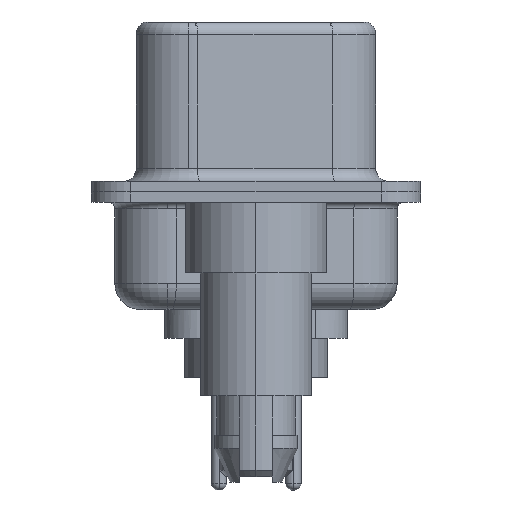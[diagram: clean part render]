
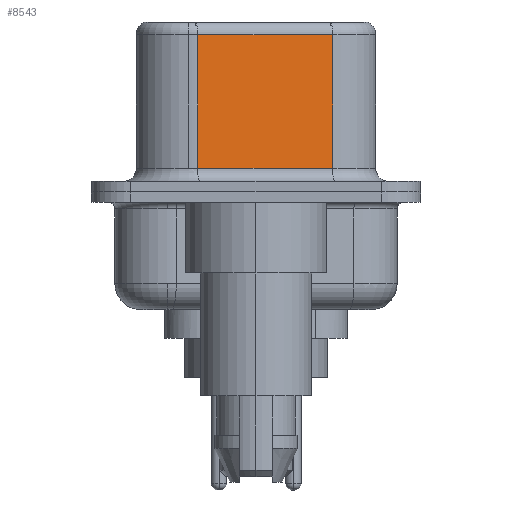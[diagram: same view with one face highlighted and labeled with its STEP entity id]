
A CAD part, left-side view. The second image highlights one B-rep face of the part: STEP entity #8543.
In plain terms, the highlighted planar face has unit normal (-0.985, -0.174, 0).
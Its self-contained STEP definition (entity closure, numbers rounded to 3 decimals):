
#245 = ORIENTED_EDGE ( 'NONE', *, *, #7230, .F. ) ;
#458 = PLANE ( 'NONE',  #13292 ) ;
#678 = VERTEX_POINT ( 'NONE', #21382 ) ;
#1195 = DIRECTION ( 'NONE',  ( 0., 0., -1. ) ) ;
#2364 = CARTESIAN_POINT ( 'NONE',  ( 4.58, -2.927, 6.02 ) ) ;
#2941 = LINE ( 'NONE', #6671, #22758 ) ;
#3120 = VECTOR ( 'NONE', #1195, 1000. ) ;
#4083 = ORIENTED_EDGE ( 'NONE', *, *, #16837, .T. ) ;
#4992 = EDGE_CURVE ( 'NONE', #20967, #20509, #14270, .T. ) ;
#5473 = DIRECTION ( 'NONE',  ( 0., 0., -1. ) ) ;
#6671 = CARTESIAN_POINT ( 'NONE',  ( 4.58, -2.927, 6.52 ) ) ;
#7089 = LINE ( 'NONE', #2364, #20712 ) ;
#7230 = EDGE_CURVE ( 'NONE', #678, #20509, #2941, .T. ) ;
#8213 = LINE ( 'NONE', #23555, #3120 ) ;
#8543 = ADVANCED_FACE ( 'NONE', ( #9182 ), #458, .F. ) ;
#9182 = FACE_OUTER_BOUND ( 'NONE', #14926, .T. ) ;
#9293 = VECTOR ( 'NONE', #22135, 1000. ) ;
#9952 = CARTESIAN_POINT ( 'NONE',  ( 4.58, -2.927, 6.52 ) ) ;
#10033 = DIRECTION ( 'NONE',  ( 0.985, 0.174, 0. ) ) ;
#10299 = EDGE_CURVE ( 'NONE', #10715, #20967, #8213, .T. ) ;
#10715 = VERTEX_POINT ( 'NONE', #14763 ) ;
#13292 = AXIS2_PLACEMENT_3D ( 'NONE', #9952, #10033, #22908 ) ;
#14270 = LINE ( 'NONE', #17908, #9293 ) ;
#14763 = CARTESIAN_POINT ( 'NONE',  ( 3.67, 2.233, 6.02 ) ) ;
#14926 = EDGE_LOOP ( 'NONE', ( #245, #4083, #22402, #20873 ) ) ;
#16837 = EDGE_CURVE ( 'NONE', #678, #10715, #7089, .T. ) ;
#17908 = CARTESIAN_POINT ( 'NONE',  ( 4.58, -2.927, 0.9 ) ) ;
#18236 = CARTESIAN_POINT ( 'NONE',  ( 4.58, -2.927, 0.9 ) ) ;
#20509 = VERTEX_POINT ( 'NONE', #18236 ) ;
#20712 = VECTOR ( 'NONE', #22918, 1000. ) ;
#20873 = ORIENTED_EDGE ( 'NONE', *, *, #4992, .T. ) ;
#20967 = VERTEX_POINT ( 'NONE', #21433 ) ;
#21382 = CARTESIAN_POINT ( 'NONE',  ( 4.58, -2.927, 6.02 ) ) ;
#21433 = CARTESIAN_POINT ( 'NONE',  ( 3.67, 2.233, 0.9 ) ) ;
#22135 = DIRECTION ( 'NONE',  ( 0.174, -0.985, 0. ) ) ;
#22402 = ORIENTED_EDGE ( 'NONE', *, *, #10299, .T. ) ;
#22758 = VECTOR ( 'NONE', #5473, 1000. ) ;
#22908 = DIRECTION ( 'NONE',  ( -0.174, 0.985, 0. ) ) ;
#22918 = DIRECTION ( 'NONE',  ( -0.174, 0.985, 0. ) ) ;
#23555 = CARTESIAN_POINT ( 'NONE',  ( 3.67, 2.233, 6.52 ) ) ;
